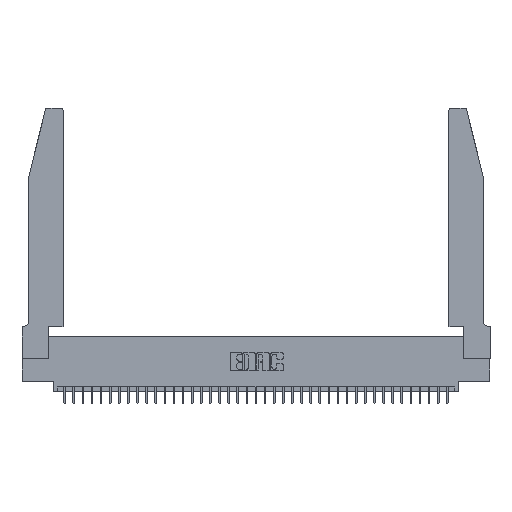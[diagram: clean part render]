
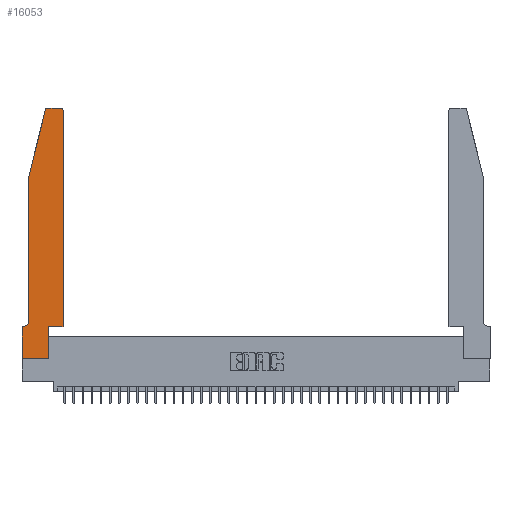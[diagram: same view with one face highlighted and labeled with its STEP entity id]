
A CAD part, top view. The second image highlights one B-rep face of the part: STEP entity #16053.
In plain terms, the highlighted planar face has unit normal (0, 0, 1).
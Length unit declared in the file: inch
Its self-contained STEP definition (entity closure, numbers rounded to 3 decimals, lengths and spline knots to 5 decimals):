
#32 = EDGE_CURVE ( 'NONE', #8187, #4928, #32753, .T. ) ;
#125 = CARTESIAN_POINT ( 'NONE',  ( 0., 0.35, 0.37 ) ) ;
#500 = AXIS2_PLACEMENT_3D ( 'NONE', #29505, #34689, #1650 ) ;
#560 = DIRECTION ( 'NONE',  ( -1., 0., 0. ) ) ;
#894 = CARTESIAN_POINT ( 'NONE',  ( 0.2865, 0., 0.37 ) ) ;
#1381 = VERTEX_POINT ( 'NONE', #12720 ) ;
#1650 = DIRECTION ( 'NONE',  ( -1., 0., 0. ) ) ;
#1768 = DIRECTION ( 'NONE',  ( -0.239, -0.971, 0. ) ) ;
#2095 = CARTESIAN_POINT ( 'NONE',  ( 0.4505, 0.35, 0.37 ) ) ;
#2810 = VECTOR ( 'NONE', #38559, 39.37008 ) ;
#3222 = ORIENTED_EDGE ( 'NONE', *, *, #27358, .T. ) ;
#4039 = CARTESIAN_POINT ( 'NONE',  ( 0.4505, 2.72, 0.37 ) ) ;
#4928 = VERTEX_POINT ( 'NONE', #36473 ) ;
#5097 = VECTOR ( 'NONE', #19650, 39.37008 ) ;
#5169 = DIRECTION ( 'NONE',  ( 1., 0., 0. ) ) ;
#5883 = CARTESIAN_POINT ( 'NONE',  ( 0., 0., 0.37 ) ) ;
#5938 = LINE ( 'NONE', #33118, #2810 ) ;
#5970 = CARTESIAN_POINT ( 'NONE',  ( 0.2865, 0.35, 0.37 ) ) ;
#7725 = CARTESIAN_POINT ( 'NONE',  ( 0.284, 2.72, 0.37 ) ) ;
#7902 = EDGE_CURVE ( 'NONE', #11149, #17874, #16656, .T. ) ;
#7916 = CARTESIAN_POINT ( 'NONE',  ( 0.4205, 2.72, 0.37 ) ) ;
#8123 = DIRECTION ( 'NONE',  ( 0., 1., 0. ) ) ;
#8187 = VERTEX_POINT ( 'NONE', #36501 ) ;
#8331 = LINE ( 'NONE', #37600, #12595 ) ;
#8804 = LINE ( 'NONE', #27362, #15536 ) ;
#9024 = VERTEX_POINT ( 'NONE', #894 ) ;
#10115 = DIRECTION ( 'NONE',  ( 1., 0., 0. ) ) ;
#10806 = ORIENTED_EDGE ( 'NONE', *, *, #31431, .T. ) ;
#11061 = CARTESIAN_POINT ( 'NONE',  ( 0.4505, 0.35, 0.37 ) ) ;
#11104 = EDGE_CURVE ( 'NONE', #22600, #15688, #36082, .T. ) ;
#11115 = AXIS2_PLACEMENT_3D ( 'NONE', #125, #35524, #29499 ) ;
#11149 = VERTEX_POINT ( 'NONE', #29045 ) ;
#11322 = ORIENTED_EDGE ( 'NONE', *, *, #36906, .T. ) ;
#11458 = CIRCLE ( 'NONE', #38278, 0.03 ) ;
#11723 = LINE ( 'NONE', #23674, #37567 ) ;
#11736 = VERTEX_POINT ( 'NONE', #4039 ) ;
#11976 = ORIENTED_EDGE ( 'NONE', *, *, #12892, .T. ) ;
#12210 = CARTESIAN_POINT ( 'NONE',  ( 0.4205, 2.75, 0.37 ) ) ;
#12595 = VECTOR ( 'NONE', #8123, 39.37008 ) ;
#12720 = CARTESIAN_POINT ( 'NONE',  ( 0.284, 2.75, 0.37 ) ) ;
#12827 = ORIENTED_EDGE ( 'NONE', *, *, #20758, .T. ) ;
#12892 = EDGE_CURVE ( 'NONE', #1381, #11149, #21045, .T. ) ;
#13394 = ORIENTED_EDGE ( 'NONE', *, *, #25725, .T. ) ;
#13687 = CARTESIAN_POINT ( 'NONE',  ( 0.0755, 0.42, 0.37 ) ) ;
#13990 = DIRECTION ( 'NONE',  ( 0., 0., 1. ) ) ;
#15408 = ORIENTED_EDGE ( 'NONE', *, *, #22763, .T. ) ;
#15536 = VECTOR ( 'NONE', #560, 39.37008 ) ;
#15688 = VERTEX_POINT ( 'NONE', #28561 ) ;
#16053 = ADVANCED_FACE ( 'NONE', ( #32604 ), #17762, .T. ) ;
#16656 = LINE ( 'NONE', #28572, #29262 ) ;
#17083 = DIRECTION ( 'NONE',  ( 1., 0., 0. ) ) ;
#17190 = VECTOR ( 'NONE', #10115, 39.37008 ) ;
#17212 = VERTEX_POINT ( 'NONE', #11061 ) ;
#17762 = PLANE ( 'NONE',  #11115 ) ;
#17874 = VERTEX_POINT ( 'NONE', #38464 ) ;
#18024 = VECTOR ( 'NONE', #35671, 39.37008 ) ;
#19650 = DIRECTION ( 'NONE',  ( 0., -1., 0. ) ) ;
#19857 = DIRECTION ( 'NONE',  ( 0., 0., 1. ) ) ;
#19874 = VERTEX_POINT ( 'NONE', #5970 ) ;
#20758 = EDGE_CURVE ( 'NONE', #4928, #9024, #31908, .T. ) ;
#21045 = CIRCLE ( 'NONE', #28557, 0.03 ) ;
#22600 = VERTEX_POINT ( 'NONE', #13687 ) ;
#22763 = EDGE_CURVE ( 'NONE', #17212, #11736, #11723, .T. ) ;
#23128 = VECTOR ( 'NONE', #17083, 39.37008 ) ;
#23387 = ORIENTED_EDGE ( 'NONE', *, *, #24545, .T. ) ;
#23674 = CARTESIAN_POINT ( 'NONE',  ( 0.4505, 0.35, 0.37 ) ) ;
#24237 = DIRECTION ( 'NONE',  ( 0., 1., 0. ) ) ;
#24545 = EDGE_CURVE ( 'NONE', #11736, #36716, #11458, .T. ) ;
#25725 = EDGE_CURVE ( 'NONE', #19874, #17212, #37642, .T. ) ;
#26901 = CARTESIAN_POINT ( 'NONE',  ( 0., 0., 0.37 ) ) ;
#27358 = EDGE_CURVE ( 'NONE', #15688, #8187, #8804, .T. ) ;
#27362 = CARTESIAN_POINT ( 'NONE',  ( 0.0755, 0.35, 0.37 ) ) ;
#27568 = ORIENTED_EDGE ( 'NONE', *, *, #32430, .T. ) ;
#28557 = AXIS2_PLACEMENT_3D ( 'NONE', #7725, #13990, #34705 ) ;
#28561 = CARTESIAN_POINT ( 'NONE',  ( 0.0055, 0.35, 0.37 ) ) ;
#28572 = CARTESIAN_POINT ( 'NONE',  ( 0.0755, 2., 0.37 ) ) ;
#29045 = CARTESIAN_POINT ( 'NONE',  ( 0.25487, 2.72718, 0.37 ) ) ;
#29262 = VECTOR ( 'NONE', #1768, 39.37008 ) ;
#29276 = ORIENTED_EDGE ( 'NONE', *, *, #11104, .T. ) ;
#29380 = ORIENTED_EDGE ( 'NONE', *, *, #7902, .T. ) ;
#29499 = DIRECTION ( 'NONE',  ( 1., 0., 0. ) ) ;
#29505 = CARTESIAN_POINT ( 'NONE',  ( 0.0055, 0.42, 0.37 ) ) ;
#31431 = EDGE_CURVE ( 'NONE', #9024, #19874, #8331, .T. ) ;
#31908 = LINE ( 'NONE', #5883, #23128 ) ;
#31959 = LINE ( 'NONE', #34296, #5097 ) ;
#32430 = EDGE_CURVE ( 'NONE', #17874, #22600, #31959, .T. ) ;
#32604 = FACE_OUTER_BOUND ( 'NONE', #37269, .T. ) ;
#32753 = LINE ( 'NONE', #26901, #18024 ) ;
#33118 = CARTESIAN_POINT ( 'NONE',  ( 0.2605, 2.75, 0.37 ) ) ;
#34296 = CARTESIAN_POINT ( 'NONE',  ( 0.0755, 2., 0.37 ) ) ;
#34689 = DIRECTION ( 'NONE',  ( 0., 0., -1. ) ) ;
#34705 = DIRECTION ( 'NONE',  ( 1., 0., 0. ) ) ;
#34795 = ORIENTED_EDGE ( 'NONE', *, *, #32, .T. ) ;
#35524 = DIRECTION ( 'NONE',  ( 0., 0., 1. ) ) ;
#35671 = DIRECTION ( 'NONE',  ( 0., -1., 0. ) ) ;
#36082 = CIRCLE ( 'NONE', #500, 0.07 ) ;
#36473 = CARTESIAN_POINT ( 'NONE',  ( 0., 0., 0.37 ) ) ;
#36501 = CARTESIAN_POINT ( 'NONE',  ( 0., 0.35, 0.37 ) ) ;
#36716 = VERTEX_POINT ( 'NONE', #12210 ) ;
#36906 = EDGE_CURVE ( 'NONE', #36716, #1381, #5938, .T. ) ;
#37269 = EDGE_LOOP ( 'NONE', ( #11322, #11976, #29380, #27568, #29276, #3222, #34795, #12827, #10806, #13394, #15408, #23387 ) ) ;
#37567 = VECTOR ( 'NONE', #24237, 39.37008 ) ;
#37600 = CARTESIAN_POINT ( 'NONE',  ( 0.2865, 0.35, 0.37 ) ) ;
#37642 = LINE ( 'NONE', #2095, #17190 ) ;
#38278 = AXIS2_PLACEMENT_3D ( 'NONE', #7916, #19857, #5169 ) ;
#38464 = CARTESIAN_POINT ( 'NONE',  ( 0.0755, 2., 0.37 ) ) ;
#38559 = DIRECTION ( 'NONE',  ( -1., 0., 0. ) ) ;
